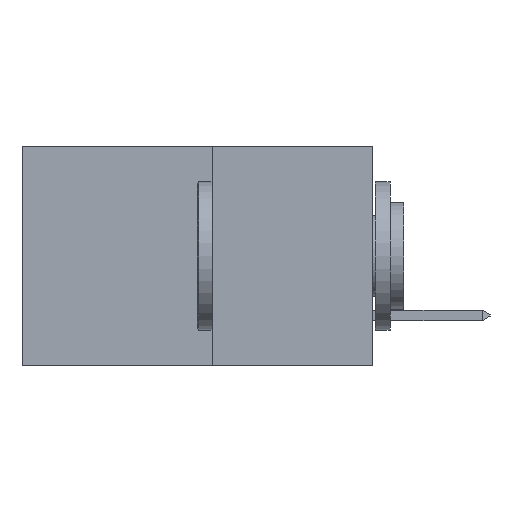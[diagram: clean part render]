
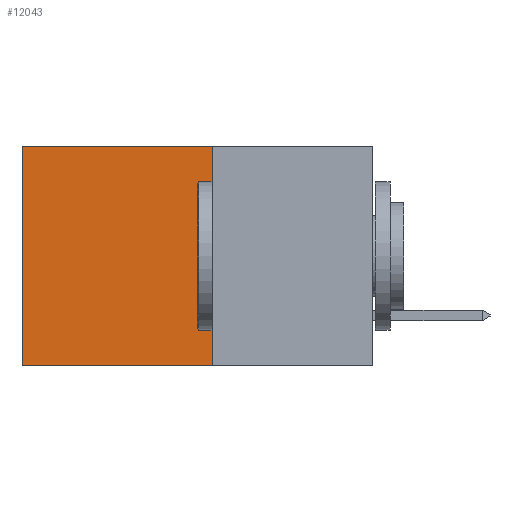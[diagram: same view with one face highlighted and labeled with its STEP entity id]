
A CAD part, left-side view. The second image highlights one B-rep face of the part: STEP entity #12043.
In plain terms, the highlighted planar face has unit normal (-1, 0, 0).
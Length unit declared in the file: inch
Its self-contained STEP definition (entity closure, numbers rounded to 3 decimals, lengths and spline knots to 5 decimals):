
#288 = ORIENTED_EDGE ( 'NONE', *, *, #15142, .F. ) ;
#2836 = CARTESIAN_POINT ( 'NONE',  ( 0.277, 0.59, 0. ) ) ;
#3174 = EDGE_CURVE ( 'NONE', #9715, #21594, #10360, .T. ) ;
#3633 = DIRECTION ( 'NONE',  ( 0., 0., -1. ) ) ;
#4172 = DIRECTION ( 'NONE',  ( 0., 1., 0. ) ) ;
#4517 = EDGE_LOOP ( 'NONE', ( #22416, #288, #8359, #9267 ) ) ;
#4577 = CARTESIAN_POINT ( 'NONE',  ( 0.277, 0.27, -0.37 ) ) ;
#6571 = CARTESIAN_POINT ( 'NONE',  ( 0.277, 0.59, -0.37 ) ) ;
#6810 = VERTEX_POINT ( 'NONE', #2836 ) ;
#6882 = LINE ( 'NONE', #18028, #11479 ) ;
#7468 = CARTESIAN_POINT ( 'NONE',  ( 0.277, 0.27, -0.37 ) ) ;
#8123 = EDGE_CURVE ( 'NONE', #9715, #6810, #13676, .T. ) ;
#8359 = ORIENTED_EDGE ( 'NONE', *, *, #3174, .F. ) ;
#8739 = VECTOR ( 'NONE', #3633, 39.37008 ) ;
#9068 = VECTOR ( 'NONE', #14375, 39.37008 ) ;
#9176 = VERTEX_POINT ( 'NONE', #16083 ) ;
#9204 = CARTESIAN_POINT ( 'NONE',  ( 0.277, 0.27, 0. ) ) ;
#9227 = DIRECTION ( 'NONE',  ( 0., 0., -1. ) ) ;
#9267 = ORIENTED_EDGE ( 'NONE', *, *, #8123, .T. ) ;
#9715 = VERTEX_POINT ( 'NONE', #9204 ) ;
#9951 = CARTESIAN_POINT ( 'NONE',  ( 0.277, 0.27, -0.37 ) ) ;
#10360 = LINE ( 'NONE', #4577, #8739 ) ;
#11479 = VECTOR ( 'NONE', #4172, 39.37008 ) ;
#12043 = ADVANCED_FACE ( 'NONE', ( #22415 ), #17804, .F. ) ;
#13676 = LINE ( 'NONE', #14699, #9068 ) ;
#14375 = DIRECTION ( 'NONE',  ( 0., 1., 0. ) ) ;
#14699 = CARTESIAN_POINT ( 'NONE',  ( 0.277, 0.27, 0. ) ) ;
#15142 = EDGE_CURVE ( 'NONE', #21594, #9176, #6882, .T. ) ;
#16083 = CARTESIAN_POINT ( 'NONE',  ( 0.277, 0.59, -0.37 ) ) ;
#16166 = VECTOR ( 'NONE', #16928, 39.37008 ) ;
#16928 = DIRECTION ( 'NONE',  ( 0., 0., -1. ) ) ;
#17229 = LINE ( 'NONE', #6571, #16166 ) ;
#17804 = PLANE ( 'NONE',  #18454 ) ;
#18028 = CARTESIAN_POINT ( 'NONE',  ( 0.277, 0.27, -0.37 ) ) ;
#18454 = AXIS2_PLACEMENT_3D ( 'NONE', #7468, #19575, #9227 ) ;
#18730 = EDGE_CURVE ( 'NONE', #6810, #9176, #17229, .T. ) ;
#19575 = DIRECTION ( 'NONE',  ( 1., 0., 0. ) ) ;
#21594 = VERTEX_POINT ( 'NONE', #9951 ) ;
#22415 = FACE_OUTER_BOUND ( 'NONE', #4517, .T. ) ;
#22416 = ORIENTED_EDGE ( 'NONE', *, *, #18730, .T. ) ;
